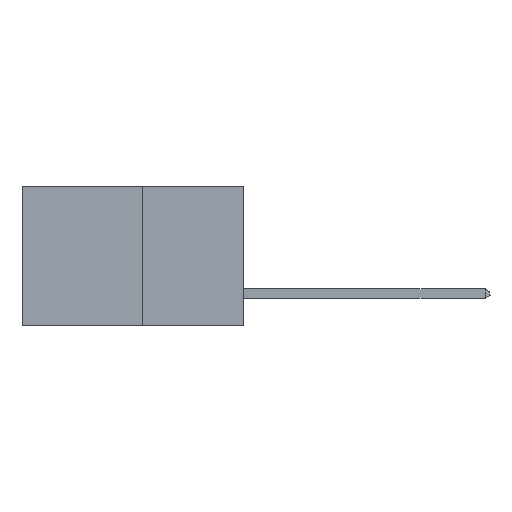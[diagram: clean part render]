
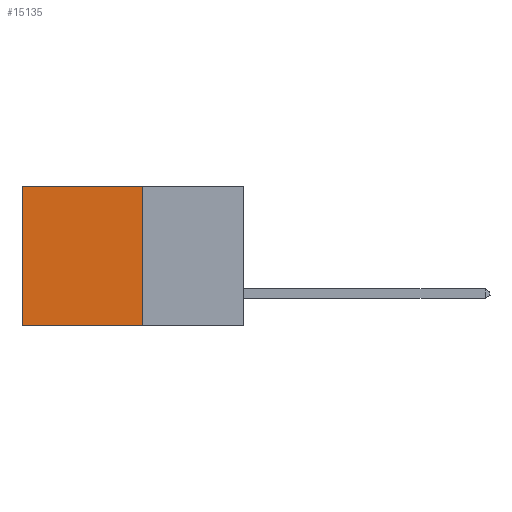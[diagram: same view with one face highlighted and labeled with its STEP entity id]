
A CAD part, left-side view. The second image highlights one B-rep face of the part: STEP entity #15135.
In plain terms, the highlighted planar face has unit normal (-1, 0, 0).
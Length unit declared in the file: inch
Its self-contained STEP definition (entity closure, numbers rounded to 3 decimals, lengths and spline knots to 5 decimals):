
#35 = DIRECTION ( 'NONE',  ( 0., 0., -1. ) ) ;
#662 = LINE ( 'NONE', #8834, #7312 ) ;
#932 = EDGE_CURVE ( 'NONE', #8797, #8729, #5116, .T. ) ;
#1060 = ORIENTED_EDGE ( 'NONE', *, *, #11953, .T. ) ;
#1474 = LINE ( 'NONE', #13223, #4345 ) ;
#1831 = PLANE ( 'NONE',  #3105 ) ;
#3072 = DIRECTION ( 'NONE',  ( 0., 0., -1. ) ) ;
#3105 = AXIS2_PLACEMENT_3D ( 'NONE', #13774, #10417, #3072 ) ;
#3211 = LINE ( 'NONE', #5534, #12450 ) ;
#4345 = VECTOR ( 'NONE', #14347, 39.37008 ) ;
#4650 = EDGE_CURVE ( 'NONE', #8797, #13211, #662, .T. ) ;
#5116 = LINE ( 'NONE', #14327, #13848 ) ;
#5534 = CARTESIAN_POINT ( 'NONE',  ( 0.277, 0.59, -0.37 ) ) ;
#7312 = VECTOR ( 'NONE', #7991, 39.37008 ) ;
#7389 = CARTESIAN_POINT ( 'NONE',  ( 0.277, 0.27, 0. ) ) ;
#7991 = DIRECTION ( 'NONE',  ( 0., 1., 0. ) ) ;
#8337 = VERTEX_POINT ( 'NONE', #13565 ) ;
#8729 = VERTEX_POINT ( 'NONE', #9722 ) ;
#8797 = VERTEX_POINT ( 'NONE', #7389 ) ;
#8834 = CARTESIAN_POINT ( 'NONE',  ( 0.277, 0.27, 0. ) ) ;
#9477 = ORIENTED_EDGE ( 'NONE', *, *, #932, .F. ) ;
#9722 = CARTESIAN_POINT ( 'NONE',  ( 0.277, 0.27, -0.37 ) ) ;
#10173 = ORIENTED_EDGE ( 'NONE', *, *, #4650, .T. ) ;
#10417 = DIRECTION ( 'NONE',  ( 1., 0., 0. ) ) ;
#11555 = DIRECTION ( 'NONE',  ( 0., 0., -1. ) ) ;
#11953 = EDGE_CURVE ( 'NONE', #13211, #8337, #3211, .T. ) ;
#12010 = CARTESIAN_POINT ( 'NONE',  ( 0.277, 0.59, 0. ) ) ;
#12253 = EDGE_CURVE ( 'NONE', #8729, #8337, #1474, .T. ) ;
#12450 = VECTOR ( 'NONE', #11555, 39.37008 ) ;
#12682 = FACE_OUTER_BOUND ( 'NONE', #12887, .T. ) ;
#12887 = EDGE_LOOP ( 'NONE', ( #1060, #12925, #9477, #10173 ) ) ;
#12925 = ORIENTED_EDGE ( 'NONE', *, *, #12253, .F. ) ;
#13211 = VERTEX_POINT ( 'NONE', #12010 ) ;
#13223 = CARTESIAN_POINT ( 'NONE',  ( 0.277, 0.27, -0.37 ) ) ;
#13565 = CARTESIAN_POINT ( 'NONE',  ( 0.277, 0.59, -0.37 ) ) ;
#13774 = CARTESIAN_POINT ( 'NONE',  ( 0.277, 0.27, -0.37 ) ) ;
#13848 = VECTOR ( 'NONE', #35, 39.37008 ) ;
#14327 = CARTESIAN_POINT ( 'NONE',  ( 0.277, 0.27, -0.37 ) ) ;
#14347 = DIRECTION ( 'NONE',  ( 0., 1., 0. ) ) ;
#15135 = ADVANCED_FACE ( 'NONE', ( #12682 ), #1831, .F. ) ;
